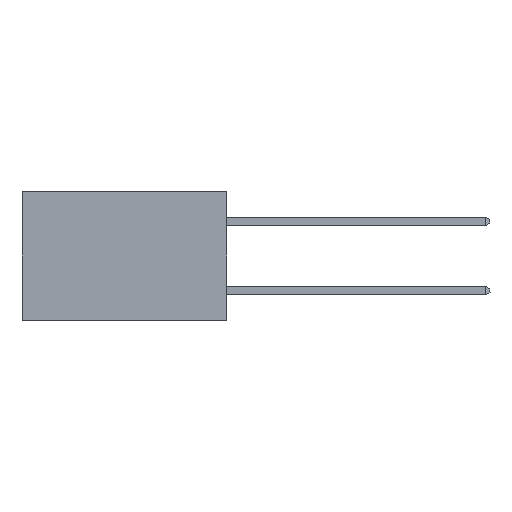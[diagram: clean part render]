
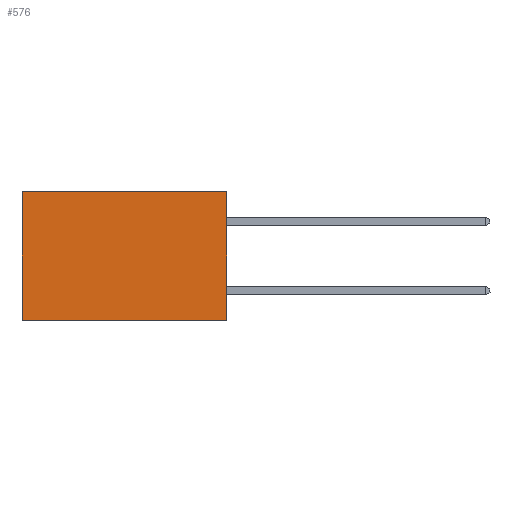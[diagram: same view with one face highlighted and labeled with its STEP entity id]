
A CAD part, left-side view. The second image highlights one B-rep face of the part: STEP entity #576.
In plain terms, the highlighted planar face has unit normal (-1, 0, 0).
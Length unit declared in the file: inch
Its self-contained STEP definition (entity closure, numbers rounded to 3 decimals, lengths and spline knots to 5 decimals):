
#277 = LINE ( 'NONE', #1671, #6212 ) ;
#576 = ADVANCED_FACE ( 'NONE', ( #8483 ), #7153, .F. ) ;
#812 = VERTEX_POINT ( 'NONE', #1166 ) ;
#1166 = CARTESIAN_POINT ( 'NONE',  ( 0.277, 0.59, -0.37 ) ) ;
#1292 = VECTOR ( 'NONE', #4925, 39.37008 ) ;
#1414 = ORIENTED_EDGE ( 'NONE', *, *, #6270, .F. ) ;
#1471 = ORIENTED_EDGE ( 'NONE', *, *, #3394, .F. ) ;
#1671 = CARTESIAN_POINT ( 'NONE',  ( 0.277, 0., -0.37 ) ) ;
#1828 = VERTEX_POINT ( 'NONE', #3373 ) ;
#1889 = ORIENTED_EDGE ( 'NONE', *, *, #4342, .T. ) ;
#1966 = VERTEX_POINT ( 'NONE', #5656 ) ;
#2275 = AXIS2_PLACEMENT_3D ( 'NONE', #2662, #7074, #4568 ) ;
#2377 = DIRECTION ( 'NONE',  ( 0., 1., 0. ) ) ;
#2662 = CARTESIAN_POINT ( 'NONE',  ( 0.277, 0., -0.37 ) ) ;
#2768 = ORIENTED_EDGE ( 'NONE', *, *, #6122, .T. ) ;
#3373 = CARTESIAN_POINT ( 'NONE',  ( 0.277, 0.59, 0. ) ) ;
#3394 = EDGE_CURVE ( 'NONE', #1966, #7218, #5279, .T. ) ;
#3410 = CARTESIAN_POINT ( 'NONE',  ( 0.277, 0.59, -0.37 ) ) ;
#4342 = EDGE_CURVE ( 'NONE', #1966, #1828, #7054, .T. ) ;
#4568 = DIRECTION ( 'NONE',  ( 0., 0., -1. ) ) ;
#4575 = EDGE_LOOP ( 'NONE', ( #2768, #1414, #1471, #1889 ) ) ;
#4874 = CARTESIAN_POINT ( 'NONE',  ( 0.277, 0., 0. ) ) ;
#4925 = DIRECTION ( 'NONE',  ( 0., 0., -1. ) ) ;
#5041 = VECTOR ( 'NONE', #8375, 39.37008 ) ;
#5247 = VECTOR ( 'NONE', #5851, 39.37008 ) ;
#5279 = LINE ( 'NONE', #8465, #5041 ) ;
#5535 = LINE ( 'NONE', #3410, #1292 ) ;
#5656 = CARTESIAN_POINT ( 'NONE',  ( 0.277, 0., 0. ) ) ;
#5851 = DIRECTION ( 'NONE',  ( 0., 1., 0. ) ) ;
#6122 = EDGE_CURVE ( 'NONE', #1828, #812, #5535, .T. ) ;
#6212 = VECTOR ( 'NONE', #2377, 39.37008 ) ;
#6270 = EDGE_CURVE ( 'NONE', #7218, #812, #277, .T. ) ;
#7047 = CARTESIAN_POINT ( 'NONE',  ( 0.277, 0., -0.37 ) ) ;
#7054 = LINE ( 'NONE', #4874, #5247 ) ;
#7074 = DIRECTION ( 'NONE',  ( 1., 0., 0. ) ) ;
#7153 = PLANE ( 'NONE',  #2275 ) ;
#7218 = VERTEX_POINT ( 'NONE', #7047 ) ;
#8375 = DIRECTION ( 'NONE',  ( 0., 0., -1. ) ) ;
#8465 = CARTESIAN_POINT ( 'NONE',  ( 0.277, 0., -0.37 ) ) ;
#8483 = FACE_OUTER_BOUND ( 'NONE', #4575, .T. ) ;
